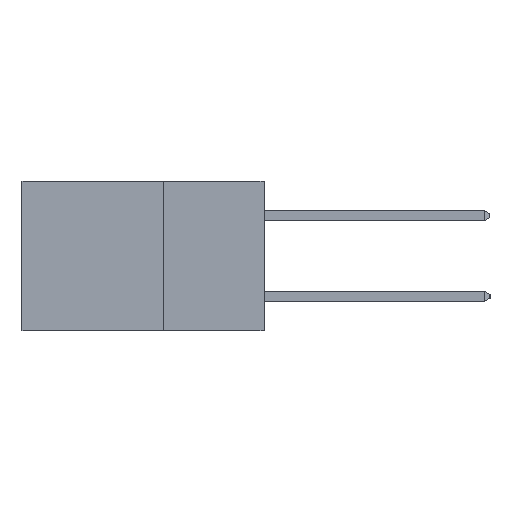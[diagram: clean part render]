
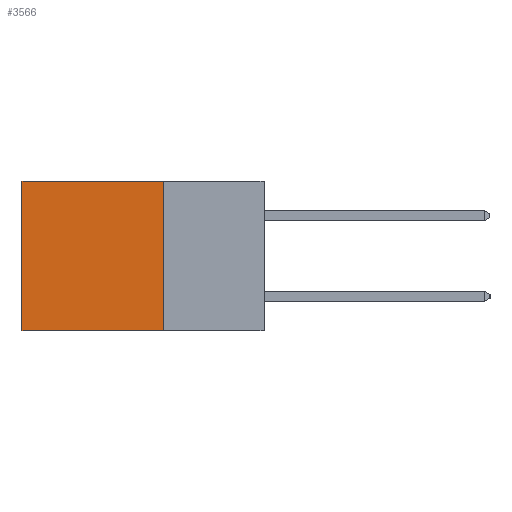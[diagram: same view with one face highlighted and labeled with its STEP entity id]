
A CAD part, left-side view. The second image highlights one B-rep face of the part: STEP entity #3566.
In plain terms, the highlighted planar face has unit normal (-1, 0, 0).
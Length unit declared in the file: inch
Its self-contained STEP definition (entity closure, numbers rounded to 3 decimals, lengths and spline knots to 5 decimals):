
#30 = LINE ( 'NONE', #1784, #4334 ) ;
#41 = CARTESIAN_POINT ( 'NONE',  ( 0.2615, 0.6, -0.37 ) ) ;
#393 = CARTESIAN_POINT ( 'NONE',  ( 0.2615, 0.25, 0. ) ) ;
#452 = DIRECTION ( 'NONE',  ( 0., 0., -1. ) ) ;
#647 = LINE ( 'NONE', #393, #6148 ) ;
#793 = VERTEX_POINT ( 'NONE', #6868 ) ;
#1198 = AXIS2_PLACEMENT_3D ( 'NONE', #7072, #5241, #452 ) ;
#1261 = EDGE_CURVE ( 'NONE', #793, #5730, #647, .T. ) ;
#1552 = EDGE_CURVE ( 'NONE', #5730, #3435, #7446, .T. ) ;
#1713 = ORIENTED_EDGE ( 'NONE', *, *, #1552, .T. ) ;
#1784 = CARTESIAN_POINT ( 'NONE',  ( 0.2615, 0.25, -0.37 ) ) ;
#2076 = LINE ( 'NONE', #4601, #4018 ) ;
#2276 = EDGE_LOOP ( 'NONE', ( #1713, #2626, #5458, #2286 ) ) ;
#2286 = ORIENTED_EDGE ( 'NONE', *, *, #1261, .T. ) ;
#2565 = EDGE_CURVE ( 'NONE', #7248, #3435, #2076, .T. ) ;
#2626 = ORIENTED_EDGE ( 'NONE', *, *, #2565, .F. ) ;
#2669 = DIRECTION ( 'NONE',  ( 0., 0., -1. ) ) ;
#2773 = CARTESIAN_POINT ( 'NONE',  ( 0.2615, 0.6, -0.37 ) ) ;
#3041 = DIRECTION ( 'NONE',  ( 0., 0., -1. ) ) ;
#3216 = FACE_OUTER_BOUND ( 'NONE', #2276, .T. ) ;
#3402 = EDGE_CURVE ( 'NONE', #793, #7248, #30, .T. ) ;
#3435 = VERTEX_POINT ( 'NONE', #2773 ) ;
#3566 = ADVANCED_FACE ( 'NONE', ( #3216 ), #8817, .F. ) ;
#4018 = VECTOR ( 'NONE', #6407, 39.37008 ) ;
#4334 = VECTOR ( 'NONE', #2669, 39.37008 ) ;
#4458 = DIRECTION ( 'NONE',  ( 0., 1., 0. ) ) ;
#4601 = CARTESIAN_POINT ( 'NONE',  ( 0.2615, 0.25, -0.37 ) ) ;
#5241 = DIRECTION ( 'NONE',  ( 1., 0., 0. ) ) ;
#5458 = ORIENTED_EDGE ( 'NONE', *, *, #3402, .F. ) ;
#5596 = VECTOR ( 'NONE', #3041, 39.37008 ) ;
#5730 = VERTEX_POINT ( 'NONE', #5996 ) ;
#5996 = CARTESIAN_POINT ( 'NONE',  ( 0.2615, 0.6, 0. ) ) ;
#6148 = VECTOR ( 'NONE', #4458, 39.37008 ) ;
#6407 = DIRECTION ( 'NONE',  ( 0., 1., 0. ) ) ;
#6868 = CARTESIAN_POINT ( 'NONE',  ( 0.2615, 0.25, 0. ) ) ;
#7072 = CARTESIAN_POINT ( 'NONE',  ( 0.2615, 0.25, -0.37 ) ) ;
#7248 = VERTEX_POINT ( 'NONE', #7757 ) ;
#7446 = LINE ( 'NONE', #41, #5596 ) ;
#7757 = CARTESIAN_POINT ( 'NONE',  ( 0.2615, 0.25, -0.37 ) ) ;
#8817 = PLANE ( 'NONE',  #1198 ) ;
